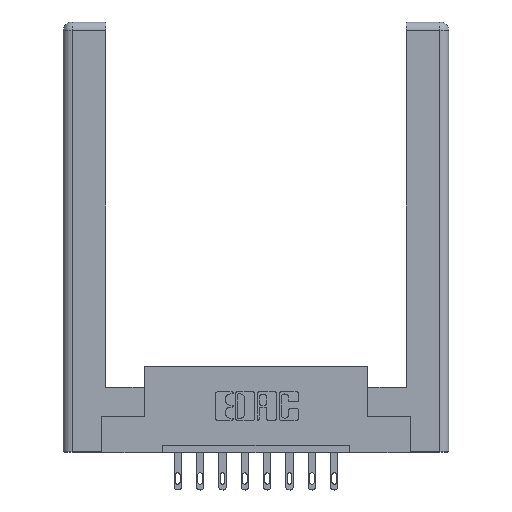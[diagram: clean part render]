
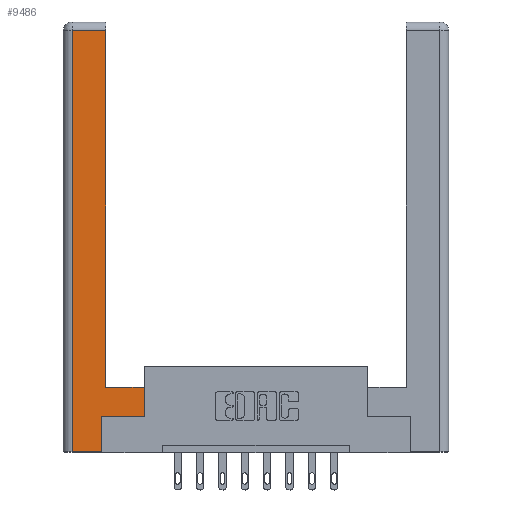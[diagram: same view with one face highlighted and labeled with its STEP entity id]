
A CAD part, top view. The second image highlights one B-rep face of the part: STEP entity #9486.
In plain terms, the highlighted planar face has unit normal (0, 0, 1).
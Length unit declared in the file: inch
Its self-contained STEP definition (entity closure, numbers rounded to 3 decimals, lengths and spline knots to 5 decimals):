
#478 = EDGE_CURVE ( 'NONE', #6401, #8917, #2889, .T. ) ;
#598 = CARTESIAN_POINT ( 'NONE',  ( 0.565, 0.245, 0. ) ) ;
#639 = LINE ( 'NONE', #598, #4429 ) ;
#657 = CARTESIAN_POINT ( 'NONE',  ( 0.265, 0.245, 0. ) ) ;
#1008 = ORIENTED_EDGE ( 'NONE', *, *, #2069, .T. ) ;
#1095 = ORIENTED_EDGE ( 'NONE', *, *, #10071, .T. ) ;
#1312 = LINE ( 'NONE', #7419, #6657 ) ;
#1315 = FACE_OUTER_BOUND ( 'NONE', #5333, .T. ) ;
#1328 = PLANE ( 'NONE',  #12095 ) ;
#2069 = EDGE_CURVE ( 'NONE', #10663, #6870, #5973, .T. ) ;
#2088 = CARTESIAN_POINT ( 'NONE',  ( 0.0615, 0., 0. ) ) ;
#2199 = CARTESIAN_POINT ( 'NONE',  ( 0.0615, 2.94, 0. ) ) ;
#2310 = EDGE_CURVE ( 'NONE', #6870, #5271, #639, .T. ) ;
#2889 = LINE ( 'NONE', #10849, #6343 ) ;
#3347 = DIRECTION ( 'NONE',  ( -1., 0., 0. ) ) ;
#3363 = ORIENTED_EDGE ( 'NONE', *, *, #10247, .T. ) ;
#3542 = CARTESIAN_POINT ( 'NONE',  ( 0.0615, 2.94, 0. ) ) ;
#3569 = VERTEX_POINT ( 'NONE', #2199 ) ;
#3958 = DIRECTION ( 'NONE',  ( -1., 0., 0. ) ) ;
#4299 = VECTOR ( 'NONE', #6576, 39.37008 ) ;
#4310 = DIRECTION ( 'NONE',  ( 0., 1., 0. ) ) ;
#4347 = CARTESIAN_POINT ( 'NONE',  ( 0.265, 0., 0. ) ) ;
#4429 = VECTOR ( 'NONE', #5815, 39.37008 ) ;
#4512 = DIRECTION ( 'NONE',  ( 1., 0., 0. ) ) ;
#4675 = CARTESIAN_POINT ( 'NONE',  ( 0.295, 2.94, 0. ) ) ;
#4679 = ORIENTED_EDGE ( 'NONE', *, *, #10178, .T. ) ;
#5204 = ORIENTED_EDGE ( 'NONE', *, *, #478, .T. ) ;
#5271 = VERTEX_POINT ( 'NONE', #11831 ) ;
#5333 = EDGE_LOOP ( 'NONE', ( #1095, #3363, #12357, #4679, #1008, #9115, #12610, #5204 ) ) ;
#5751 = DIRECTION ( 'NONE',  ( 0., 1., 0. ) ) ;
#5815 = DIRECTION ( 'NONE',  ( 1., 0., 0. ) ) ;
#5973 = LINE ( 'NONE', #7680, #11907 ) ;
#6335 = LINE ( 'NONE', #3542, #4299 ) ;
#6343 = VECTOR ( 'NONE', #3958, 39.37008 ) ;
#6348 = VECTOR ( 'NONE', #7130, 39.37008 ) ;
#6401 = VERTEX_POINT ( 'NONE', #12692 ) ;
#6576 = DIRECTION ( 'NONE',  ( -1., 0., 0. ) ) ;
#6657 = VECTOR ( 'NONE', #12474, 39.37008 ) ;
#6870 = VERTEX_POINT ( 'NONE', #657 ) ;
#7130 = DIRECTION ( 'NONE',  ( 0., -1., 0. ) ) ;
#7245 = EDGE_CURVE ( 'NONE', #5271, #6401, #1312, .T. ) ;
#7419 = CARTESIAN_POINT ( 'NONE',  ( 0.565, 0.45, 0. ) ) ;
#7680 = CARTESIAN_POINT ( 'NONE',  ( 0.265, 0.245, 0. ) ) ;
#8051 = LINE ( 'NONE', #10283, #6348 ) ;
#8426 = DIRECTION ( 'NONE',  ( 0., 0., -1. ) ) ;
#8600 = VERTEX_POINT ( 'NONE', #4675 ) ;
#8917 = VERTEX_POINT ( 'NONE', #10991 ) ;
#9115 = ORIENTED_EDGE ( 'NONE', *, *, #2310, .T. ) ;
#9269 = VECTOR ( 'NONE', #4512, 39.37008 ) ;
#9402 = CARTESIAN_POINT ( 'NONE',  ( 0., 0., 0. ) ) ;
#9409 = EDGE_CURVE ( 'NONE', #3569, #12235, #8051, .T. ) ;
#9486 = ADVANCED_FACE ( 'NONE', ( #1315 ), #1328, .F. ) ;
#10071 = EDGE_CURVE ( 'NONE', #8917, #8600, #11938, .T. ) ;
#10178 = EDGE_CURVE ( 'NONE', #12235, #10663, #10831, .T. ) ;
#10230 = VECTOR ( 'NONE', #4310, 39.37008 ) ;
#10247 = EDGE_CURVE ( 'NONE', #8600, #3569, #6335, .T. ) ;
#10271 = CARTESIAN_POINT ( 'NONE',  ( 0.295, 3., 0. ) ) ;
#10283 = CARTESIAN_POINT ( 'NONE',  ( 0.0615, 0., 0. ) ) ;
#10663 = VERTEX_POINT ( 'NONE', #4347 ) ;
#10831 = LINE ( 'NONE', #11450, #9269 ) ;
#10849 = CARTESIAN_POINT ( 'NONE',  ( 0.295, 0.45, 0. ) ) ;
#10991 = CARTESIAN_POINT ( 'NONE',  ( 0.295, 0.45, 0. ) ) ;
#11450 = CARTESIAN_POINT ( 'NONE',  ( 0.265, 0., 0. ) ) ;
#11831 = CARTESIAN_POINT ( 'NONE',  ( 0.565, 0.245, 0. ) ) ;
#11907 = VECTOR ( 'NONE', #5751, 39.37008 ) ;
#11938 = LINE ( 'NONE', #10271, #10230 ) ;
#12095 = AXIS2_PLACEMENT_3D ( 'NONE', #9402, #8426, #3347 ) ;
#12235 = VERTEX_POINT ( 'NONE', #2088 ) ;
#12357 = ORIENTED_EDGE ( 'NONE', *, *, #9409, .T. ) ;
#12474 = DIRECTION ( 'NONE',  ( 0., 1., 0. ) ) ;
#12610 = ORIENTED_EDGE ( 'NONE', *, *, #7245, .T. ) ;
#12692 = CARTESIAN_POINT ( 'NONE',  ( 0.565, 0.45, 0. ) ) ;
